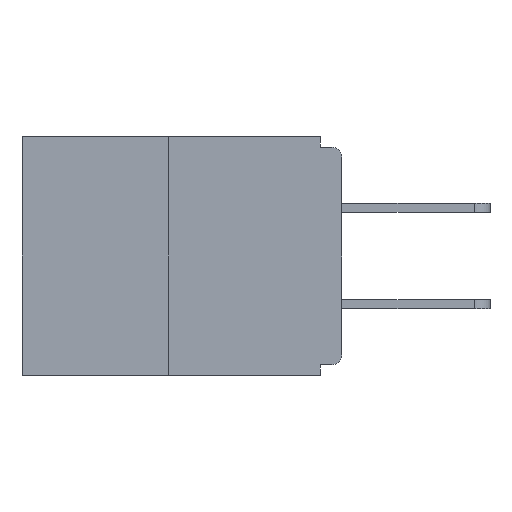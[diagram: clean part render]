
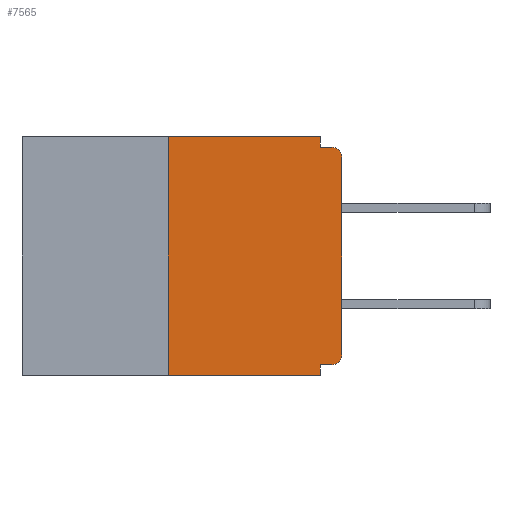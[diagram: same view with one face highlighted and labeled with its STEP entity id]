
A CAD part, left-side view. The second image highlights one B-rep face of the part: STEP entity #7565.
In plain terms, the highlighted planar face has unit normal (-1, 0, 0).
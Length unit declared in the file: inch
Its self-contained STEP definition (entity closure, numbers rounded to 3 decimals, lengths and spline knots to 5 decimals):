
#58 = AXIS2_PLACEMENT_3D ( 'NONE', #6465, #1243, #9028 ) ;
#124 = CARTESIAN_POINT ( 'NONE',  ( 0., 0.25, 0. ) ) ;
#257 = VERTEX_POINT ( 'NONE', #3321 ) ;
#282 = VECTOR ( 'NONE', #899, 39.37008 ) ;
#373 = FACE_OUTER_BOUND ( 'NONE', #7177, .T. ) ;
#493 = EDGE_CURVE ( 'NONE', #9819, #4031, #8955, .T. ) ;
#828 = ORIENTED_EDGE ( 'NONE', *, *, #9167, .T. ) ;
#860 = CARTESIAN_POINT ( 'NONE',  ( 0., 0.031, -0.328 ) ) ;
#899 = DIRECTION ( 'NONE',  ( 0., 0., -1. ) ) ;
#1027 = DIRECTION ( 'NONE',  ( 0., -1., 0. ) ) ;
#1130 = CARTESIAN_POINT ( 'NONE',  ( 0., 0.031, 0. ) ) ;
#1202 = EDGE_CURVE ( 'NONE', #1283, #257, #3144, .T. ) ;
#1243 = DIRECTION ( 'NONE',  ( -1., 0., 0. ) ) ;
#1283 = VERTEX_POINT ( 'NONE', #860 ) ;
#1346 = DIRECTION ( 'NONE',  ( 0., 1., 0. ) ) ;
#1540 = EDGE_CURVE ( 'NONE', #5960, #9819, #6115, .T. ) ;
#1896 = DIRECTION ( 'NONE',  ( 0., -1., 0. ) ) ;
#1902 = LINE ( 'NONE', #8881, #6254 ) ;
#1917 = CARTESIAN_POINT ( 'NONE',  ( 0., 0.25, 0. ) ) ;
#1919 = ORIENTED_EDGE ( 'NONE', *, *, #8670, .F. ) ;
#1995 = EDGE_CURVE ( 'NONE', #9978, #5492, #2193, .T. ) ;
#2070 = CARTESIAN_POINT ( 'NONE',  ( 0., 0.25, -0.343 ) ) ;
#2079 = VECTOR ( 'NONE', #3867, 39.37008 ) ;
#2115 = ORIENTED_EDGE ( 'NONE', *, *, #1202, .F. ) ;
#2122 = CARTESIAN_POINT ( 'NONE',  ( 0., 0., -0.328 ) ) ;
#2149 = EDGE_CURVE ( 'NONE', #8029, #257, #1902, .T. ) ;
#2193 = CIRCLE ( 'NONE', #58, 0.015 ) ;
#2262 = VECTOR ( 'NONE', #8862, 39.37008 ) ;
#2301 = ORIENTED_EDGE ( 'NONE', *, *, #2525, .F. ) ;
#2326 = ORIENTED_EDGE ( 'NONE', *, *, #493, .F. ) ;
#2347 = CARTESIAN_POINT ( 'NONE',  ( 0., 0., -0.313 ) ) ;
#2525 = EDGE_CURVE ( 'NONE', #4031, #5492, #6770, .T. ) ;
#2709 = DIRECTION ( 'NONE',  ( 0., 0., -1. ) ) ;
#3144 = LINE ( 'NONE', #5326, #282 ) ;
#3213 = VECTOR ( 'NONE', #1346, 39.37008 ) ;
#3215 = CARTESIAN_POINT ( 'NONE',  ( 0., 0.015, -0.313 ) ) ;
#3303 = ORIENTED_EDGE ( 'NONE', *, *, #1995, .T. ) ;
#3321 = CARTESIAN_POINT ( 'NONE',  ( 0., 0.031, -0.343 ) ) ;
#3620 = LINE ( 'NONE', #2122, #3213 ) ;
#3621 = ORIENTED_EDGE ( 'NONE', *, *, #8618, .T. ) ;
#3867 = DIRECTION ( 'NONE',  ( 0., 0., -1. ) ) ;
#4031 = VERTEX_POINT ( 'NONE', #10507 ) ;
#4405 = LINE ( 'NONE', #7119, #7641 ) ;
#4592 = CARTESIAN_POINT ( 'NONE',  ( 0., 0.015, -0.328 ) ) ;
#4724 = AXIS2_PLACEMENT_3D ( 'NONE', #5264, #7867, #2709 ) ;
#4893 = CARTESIAN_POINT ( 'NONE',  ( 0., 0., -0.03 ) ) ;
#4929 = DIRECTION ( 'NONE',  ( 0., 0., -1. ) ) ;
#5102 = DIRECTION ( 'NONE',  ( 0., -1., 0. ) ) ;
#5264 = CARTESIAN_POINT ( 'NONE',  ( 0., 0.46, 0. ) ) ;
#5326 = CARTESIAN_POINT ( 'NONE',  ( 0., 0.031, -0.343 ) ) ;
#5492 = VERTEX_POINT ( 'NONE', #8105 ) ;
#5553 = VECTOR ( 'NONE', #5102, 39.37008 ) ;
#5640 = AXIS2_PLACEMENT_3D ( 'NONE', #3215, #10101, #4929 ) ;
#5960 = VERTEX_POINT ( 'NONE', #124 ) ;
#6115 = LINE ( 'NONE', #6116, #7328 ) ;
#6116 = CARTESIAN_POINT ( 'NONE',  ( 0., 0.46, 0. ) ) ;
#6254 = VECTOR ( 'NONE', #1896, 39.37008 ) ;
#6309 = ORIENTED_EDGE ( 'NONE', *, *, #2149, .T. ) ;
#6334 = CIRCLE ( 'NONE', #5640, 0.015 ) ;
#6465 = CARTESIAN_POINT ( 'NONE',  ( 0., 0.015, -0.03 ) ) ;
#6770 = LINE ( 'NONE', #9505, #5553 ) ;
#6865 = LINE ( 'NONE', #1917, #2262 ) ;
#7119 = CARTESIAN_POINT ( 'NONE',  ( 0., 0., 0. ) ) ;
#7177 = EDGE_LOOP ( 'NONE', ( #10450, #8548, #6309, #2115, #1919, #828, #3621, #3303, #2301, #2326 ) ) ;
#7328 = VECTOR ( 'NONE', #1027, 39.37008 ) ;
#7565 = ADVANCED_FACE ( 'NONE', ( #373 ), #8644, .F. ) ;
#7641 = VECTOR ( 'NONE', #8835, 39.37008 ) ;
#7867 = DIRECTION ( 'NONE',  ( 1., 0., 0. ) ) ;
#8029 = VERTEX_POINT ( 'NONE', #2070 ) ;
#8055 = VERTEX_POINT ( 'NONE', #4592 ) ;
#8105 = CARTESIAN_POINT ( 'NONE',  ( 0., 0.015, -0.015 ) ) ;
#8218 = EDGE_CURVE ( 'NONE', #8029, #5960, #6865, .T. ) ;
#8548 = ORIENTED_EDGE ( 'NONE', *, *, #8218, .F. ) ;
#8618 = EDGE_CURVE ( 'NONE', #8788, #9978, #4405, .T. ) ;
#8644 = PLANE ( 'NONE',  #4724 ) ;
#8670 = EDGE_CURVE ( 'NONE', #8055, #1283, #3620, .T. ) ;
#8788 = VERTEX_POINT ( 'NONE', #2347 ) ;
#8835 = DIRECTION ( 'NONE',  ( 0., 0., 1. ) ) ;
#8862 = DIRECTION ( 'NONE',  ( 0., 0., 1. ) ) ;
#8881 = CARTESIAN_POINT ( 'NONE',  ( 0., 0.46, -0.343 ) ) ;
#8955 = LINE ( 'NONE', #9015, #2079 ) ;
#9015 = CARTESIAN_POINT ( 'NONE',  ( 0., 0.031, 0. ) ) ;
#9028 = DIRECTION ( 'NONE',  ( 0., 0., -1. ) ) ;
#9167 = EDGE_CURVE ( 'NONE', #8055, #8788, #6334, .T. ) ;
#9505 = CARTESIAN_POINT ( 'NONE',  ( 0., 0., -0.015 ) ) ;
#9819 = VERTEX_POINT ( 'NONE', #1130 ) ;
#9978 = VERTEX_POINT ( 'NONE', #4893 ) ;
#10101 = DIRECTION ( 'NONE',  ( -1., 0., 0. ) ) ;
#10450 = ORIENTED_EDGE ( 'NONE', *, *, #1540, .F. ) ;
#10507 = CARTESIAN_POINT ( 'NONE',  ( 0., 0.031, -0.015 ) ) ;
